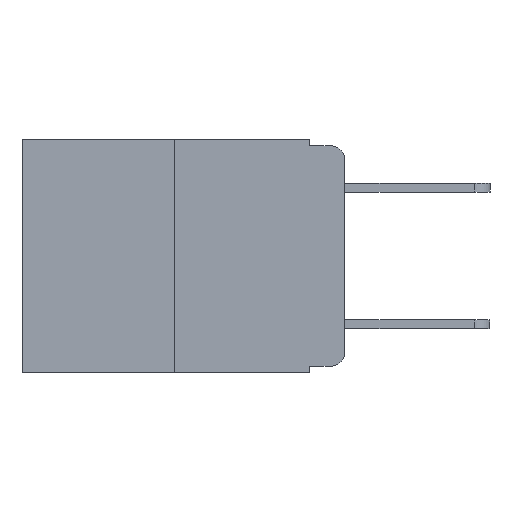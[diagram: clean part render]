
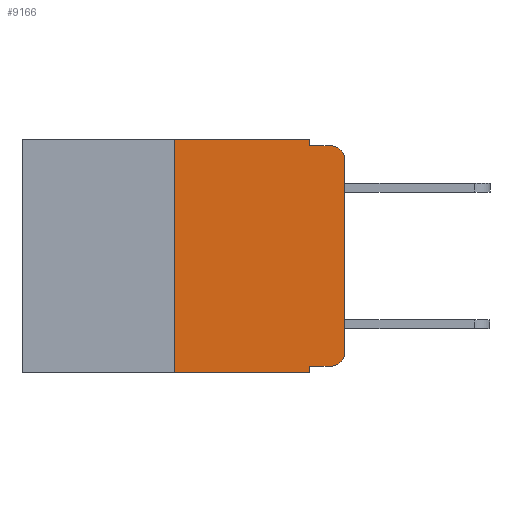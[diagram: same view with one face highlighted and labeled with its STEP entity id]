
A CAD part, left-side view. The second image highlights one B-rep face of the part: STEP entity #9166.
In plain terms, the highlighted planar face has unit normal (-1, 0, 0).
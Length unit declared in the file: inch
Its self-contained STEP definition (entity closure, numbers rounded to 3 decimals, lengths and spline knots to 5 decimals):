
#342 = EDGE_CURVE ( 'NONE', #16202, #14661, #17989, .T. ) ;
#553 = LINE ( 'NONE', #4977, #12167 ) ;
#920 = DIRECTION ( 'NONE',  ( 0., -1., 0. ) ) ;
#972 = EDGE_CURVE ( 'NONE', #16078, #13221, #17958, .T. ) ;
#991 = VECTOR ( 'NONE', #16928, 39.37008 ) ;
#1330 = CARTESIAN_POINT ( 'NONE',  ( 0., 0.051, -0.333 ) ) ;
#1431 = DIRECTION ( 'NONE',  ( 0., -1., 0. ) ) ;
#1628 = DIRECTION ( 'NONE',  ( 1., 0., 0. ) ) ;
#1746 = DIRECTION ( 'NONE',  ( 0., 0., -1. ) ) ;
#1963 = CARTESIAN_POINT ( 'NONE',  ( 0., 0.051, 0. ) ) ;
#1992 = VERTEX_POINT ( 'NONE', #7948 ) ;
#2132 = DIRECTION ( 'NONE',  ( 0., 0., 1. ) ) ;
#2193 = LINE ( 'NONE', #14367, #13532 ) ;
#2552 = ORIENTED_EDGE ( 'NONE', *, *, #7067, .F. ) ;
#2684 = CARTESIAN_POINT ( 'NONE',  ( 0., 0.051, -0.343 ) ) ;
#2788 = AXIS2_PLACEMENT_3D ( 'NONE', #10751, #1628, #12140 ) ;
#2976 = AXIS2_PLACEMENT_3D ( 'NONE', #6038, #15924, #7511 ) ;
#3181 = PLANE ( 'NONE',  #2788 ) ;
#3551 = CARTESIAN_POINT ( 'NONE',  ( 0., 0.25, 0. ) ) ;
#3822 = ORIENTED_EDGE ( 'NONE', *, *, #12890, .T. ) ;
#4506 = ORIENTED_EDGE ( 'NONE', *, *, #18445, .T. ) ;
#4977 = CARTESIAN_POINT ( 'NONE',  ( 0., 0.051, 0. ) ) ;
#5228 = LINE ( 'NONE', #13906, #15724 ) ;
#5331 = EDGE_LOOP ( 'NONE', ( #8582, #3822, #12153, #11311, #11924, #2552, #15968, #17900, #15537, #4506 ) ) ;
#5592 = CARTESIAN_POINT ( 'NONE',  ( 0., 0.051, -0.333 ) ) ;
#6038 = CARTESIAN_POINT ( 'NONE',  ( 0., 0.02, -0.03 ) ) ;
#6328 = EDGE_CURVE ( 'NONE', #1992, #18159, #5228, .T. ) ;
#6494 = EDGE_CURVE ( 'NONE', #17928, #14661, #9941, .T. ) ;
#6720 = CARTESIAN_POINT ( 'NONE',  ( 0., 0.25, -0.343 ) ) ;
#6793 = CARTESIAN_POINT ( 'NONE',  ( 0., 0., -0.03 ) ) ;
#7067 = EDGE_CURVE ( 'NONE', #17928, #15445, #9480, .T. ) ;
#7317 = EDGE_CURVE ( 'NONE', #16202, #9875, #9248, .T. ) ;
#7335 = DIRECTION ( 'NONE',  ( 0., 0., -1. ) ) ;
#7511 = DIRECTION ( 'NONE',  ( 0., 0., -1. ) ) ;
#7948 = CARTESIAN_POINT ( 'NONE',  ( 0., 0., -0.313 ) ) ;
#8170 = CARTESIAN_POINT ( 'NONE',  ( 0., 0.02, -0.01 ) ) ;
#8386 = DIRECTION ( 'NONE',  ( 0., 0., -1. ) ) ;
#8582 = ORIENTED_EDGE ( 'NONE', *, *, #6328, .T. ) ;
#9166 = ADVANCED_FACE ( 'NONE', ( #11841 ), #3181, .F. ) ;
#9248 = LINE ( 'NONE', #5592, #991 ) ;
#9369 = DIRECTION ( 'NONE',  ( -1., 0., 0. ) ) ;
#9480 = LINE ( 'NONE', #3551, #16333 ) ;
#9502 = VECTOR ( 'NONE', #920, 39.37008 ) ;
#9682 = DIRECTION ( 'NONE',  ( 0., 0., 1. ) ) ;
#9875 = VERTEX_POINT ( 'NONE', #13593 ) ;
#9941 = LINE ( 'NONE', #11560, #9502 ) ;
#10264 = CIRCLE ( 'NONE', #16469, 0.02 ) ;
#10751 = CARTESIAN_POINT ( 'NONE',  ( 0., 0.473, 0. ) ) ;
#11311 = ORIENTED_EDGE ( 'NONE', *, *, #12069, .F. ) ;
#11557 = CARTESIAN_POINT ( 'NONE',  ( 0., 0.051, -0.01 ) ) ;
#11560 = CARTESIAN_POINT ( 'NONE',  ( 0., 0.473, -0.343 ) ) ;
#11841 = FACE_OUTER_BOUND ( 'NONE', #5331, .T. ) ;
#11924 = ORIENTED_EDGE ( 'NONE', *, *, #17701, .F. ) ;
#12069 = EDGE_CURVE ( 'NONE', #17892, #16078, #553, .T. ) ;
#12140 = DIRECTION ( 'NONE',  ( 0., 0., -1. ) ) ;
#12153 = ORIENTED_EDGE ( 'NONE', *, *, #972, .F. ) ;
#12167 = VECTOR ( 'NONE', #1746, 39.37008 ) ;
#12890 = EDGE_CURVE ( 'NONE', #18159, #13221, #16823, .T. ) ;
#12991 = CARTESIAN_POINT ( 'NONE',  ( 0., 0.051, -0.01 ) ) ;
#13221 = VERTEX_POINT ( 'NONE', #8170 ) ;
#13532 = VECTOR ( 'NONE', #15728, 39.37008 ) ;
#13593 = CARTESIAN_POINT ( 'NONE',  ( 0., 0.02, -0.333 ) ) ;
#13906 = CARTESIAN_POINT ( 'NONE',  ( 0., 0., 0. ) ) ;
#13927 = CARTESIAN_POINT ( 'NONE',  ( 0., 0.25, 0. ) ) ;
#14332 = VECTOR ( 'NONE', #1431, 39.37008 ) ;
#14364 = VECTOR ( 'NONE', #8386, 39.37008 ) ;
#14367 = CARTESIAN_POINT ( 'NONE',  ( 0., 0.473, 0. ) ) ;
#14661 = VERTEX_POINT ( 'NONE', #2684 ) ;
#15445 = VERTEX_POINT ( 'NONE', #13927 ) ;
#15537 = ORIENTED_EDGE ( 'NONE', *, *, #7317, .T. ) ;
#15724 = VECTOR ( 'NONE', #2132, 39.37008 ) ;
#15728 = DIRECTION ( 'NONE',  ( 0., -1., 0. ) ) ;
#15924 = DIRECTION ( 'NONE',  ( -1., 0., 0. ) ) ;
#15968 = ORIENTED_EDGE ( 'NONE', *, *, #6494, .T. ) ;
#16078 = VERTEX_POINT ( 'NONE', #11557 ) ;
#16202 = VERTEX_POINT ( 'NONE', #1330 ) ;
#16280 = CARTESIAN_POINT ( 'NONE',  ( 0., 0.051, 0. ) ) ;
#16333 = VECTOR ( 'NONE', #9682, 39.37008 ) ;
#16469 = AXIS2_PLACEMENT_3D ( 'NONE', #17586, #9369, #7335 ) ;
#16823 = CIRCLE ( 'NONE', #2976, 0.02 ) ;
#16928 = DIRECTION ( 'NONE',  ( 0., -1., 0. ) ) ;
#17586 = CARTESIAN_POINT ( 'NONE',  ( 0., 0.02, -0.313 ) ) ;
#17701 = EDGE_CURVE ( 'NONE', #15445, #17892, #2193, .T. ) ;
#17892 = VERTEX_POINT ( 'NONE', #1963 ) ;
#17900 = ORIENTED_EDGE ( 'NONE', *, *, #342, .F. ) ;
#17928 = VERTEX_POINT ( 'NONE', #6720 ) ;
#17958 = LINE ( 'NONE', #12991, #14332 ) ;
#17989 = LINE ( 'NONE', #16280, #14364 ) ;
#18159 = VERTEX_POINT ( 'NONE', #6793 ) ;
#18445 = EDGE_CURVE ( 'NONE', #9875, #1992, #10264, .T. ) ;
